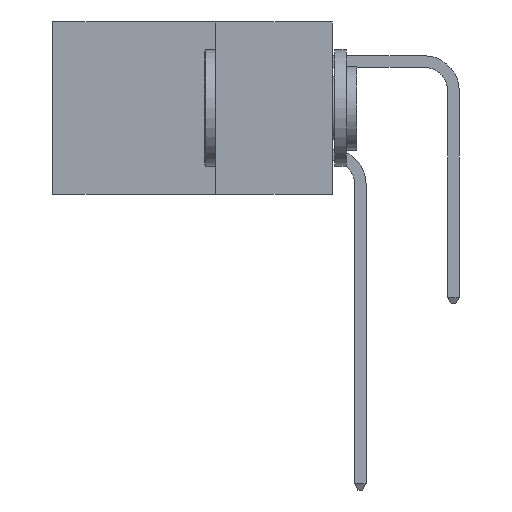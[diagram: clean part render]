
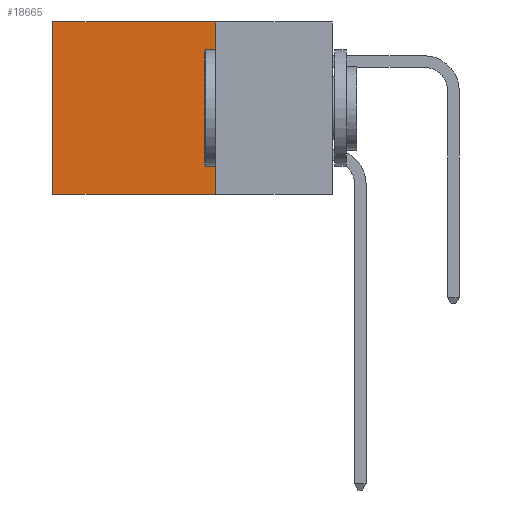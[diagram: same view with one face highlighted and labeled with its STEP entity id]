
A CAD part, left-side view. The second image highlights one B-rep face of the part: STEP entity #18665.
In plain terms, the highlighted planar face has unit normal (-1, 0, 0).
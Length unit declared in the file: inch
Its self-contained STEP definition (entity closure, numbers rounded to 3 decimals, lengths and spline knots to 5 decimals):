
#401 = DIRECTION ( 'NONE',  ( 1., 0., 0. ) ) ;
#882 = ORIENTED_EDGE ( 'NONE', *, *, #7146, .F. ) ;
#1599 = EDGE_CURVE ( 'NONE', #19950, #4025, #7219, .T. ) ;
#3101 = CARTESIAN_POINT ( 'NONE',  ( 0.2615, 0.6, -0.37 ) ) ;
#3445 = CARTESIAN_POINT ( 'NONE',  ( 0.2615, 0.6, 0. ) ) ;
#4025 = VERTEX_POINT ( 'NONE', #8361 ) ;
#4796 = EDGE_LOOP ( 'NONE', ( #10141, #882, #11017, #20137 ) ) ;
#5281 = VERTEX_POINT ( 'NONE', #11423 ) ;
#6704 = CARTESIAN_POINT ( 'NONE',  ( 0.2615, 0.25, -0.37 ) ) ;
#6762 = EDGE_CURVE ( 'NONE', #17811, #5281, #18315, .T. ) ;
#7146 = EDGE_CURVE ( 'NONE', #4025, #5281, #8250, .T. ) ;
#7204 = CARTESIAN_POINT ( 'NONE',  ( 0.2615, 0.25, 0. ) ) ;
#7219 = LINE ( 'NONE', #17126, #10898 ) ;
#8250 = LINE ( 'NONE', #13489, #16625 ) ;
#8361 = CARTESIAN_POINT ( 'NONE',  ( 0.2615, 0.25, -0.37 ) ) ;
#8782 = VECTOR ( 'NONE', #18149, 39.37008 ) ;
#9850 = PLANE ( 'NONE',  #17801 ) ;
#10141 = ORIENTED_EDGE ( 'NONE', *, *, #6762, .T. ) ;
#10898 = VECTOR ( 'NONE', #16023, 39.37008 ) ;
#11017 = ORIENTED_EDGE ( 'NONE', *, *, #1599, .F. ) ;
#11423 = CARTESIAN_POINT ( 'NONE',  ( 0.2615, 0.6, -0.37 ) ) ;
#11432 = DIRECTION ( 'NONE',  ( 0., 0., -1. ) ) ;
#13489 = CARTESIAN_POINT ( 'NONE',  ( 0.2615, 0.25, -0.37 ) ) ;
#13948 = CARTESIAN_POINT ( 'NONE',  ( 0.2615, 0.25, 0. ) ) ;
#14161 = VECTOR ( 'NONE', #18748, 39.37008 ) ;
#15078 = DIRECTION ( 'NONE',  ( 0., 1., 0. ) ) ;
#16023 = DIRECTION ( 'NONE',  ( 0., 0., -1. ) ) ;
#16625 = VECTOR ( 'NONE', #15078, 39.37008 ) ;
#16672 = LINE ( 'NONE', #7204, #8782 ) ;
#17126 = CARTESIAN_POINT ( 'NONE',  ( 0.2615, 0.25, -0.37 ) ) ;
#17548 = EDGE_CURVE ( 'NONE', #19950, #17811, #16672, .T. ) ;
#17801 = AXIS2_PLACEMENT_3D ( 'NONE', #6704, #401, #11432 ) ;
#17811 = VERTEX_POINT ( 'NONE', #3445 ) ;
#17826 = FACE_OUTER_BOUND ( 'NONE', #4796, .T. ) ;
#18149 = DIRECTION ( 'NONE',  ( 0., 1., 0. ) ) ;
#18315 = LINE ( 'NONE', #3101, #14161 ) ;
#18665 = ADVANCED_FACE ( 'NONE', ( #17826 ), #9850, .F. ) ;
#18748 = DIRECTION ( 'NONE',  ( 0., 0., -1. ) ) ;
#19950 = VERTEX_POINT ( 'NONE', #13948 ) ;
#20137 = ORIENTED_EDGE ( 'NONE', *, *, #17548, .T. ) ;
